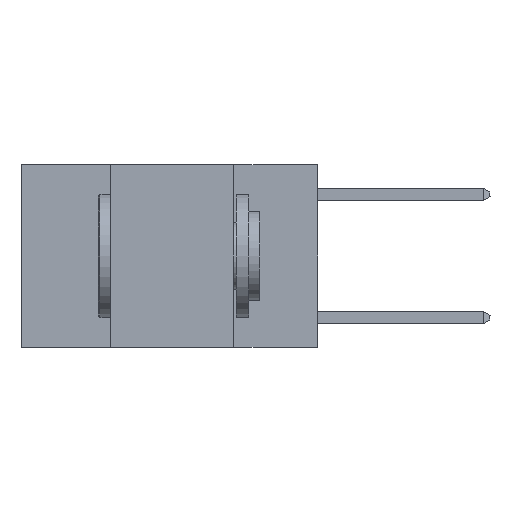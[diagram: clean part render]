
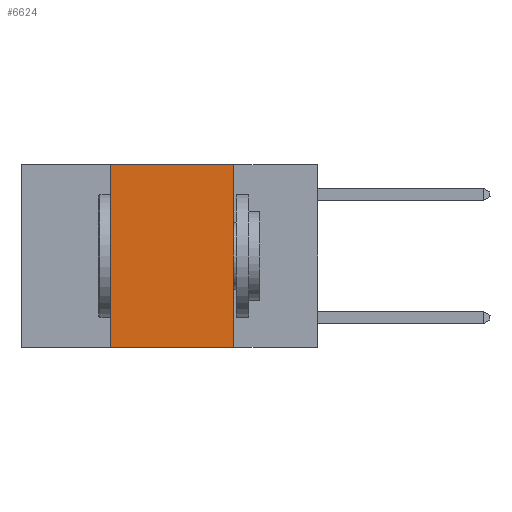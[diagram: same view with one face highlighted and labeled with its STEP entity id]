
A CAD part, left-side view. The second image highlights one B-rep face of the part: STEP entity #6624.
In plain terms, the highlighted planar face has unit normal (-1, 0, 0).
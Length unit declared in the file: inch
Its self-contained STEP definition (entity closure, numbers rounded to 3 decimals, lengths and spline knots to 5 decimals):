
#243 = VERTEX_POINT ( 'NONE', #1435 ) ;
#548 = DIRECTION ( 'NONE',  ( 0., -1., 0. ) ) ;
#835 = LINE ( 'NONE', #12542, #7269 ) ;
#889 = ORIENTED_EDGE ( 'NONE', *, *, #5118, .F. ) ;
#1435 = CARTESIAN_POINT ( 'NONE',  ( 0., 0.17, 0. ) ) ;
#1640 = DIRECTION ( 'NONE',  ( 1., 0., 0. ) ) ;
#1732 = VECTOR ( 'NONE', #548, 39.37008 ) ;
#1780 = LINE ( 'NONE', #12583, #4726 ) ;
#2160 = AXIS2_PLACEMENT_3D ( 'NONE', #2364, #1640, #7473 ) ;
#2265 = CARTESIAN_POINT ( 'NONE',  ( 0., 0.42, 0. ) ) ;
#2364 = CARTESIAN_POINT ( 'NONE',  ( 0., 0.6, 0. ) ) ;
#2411 = EDGE_CURVE ( 'NONE', #8634, #5942, #1780, .T. ) ;
#2758 = LINE ( 'NONE', #9240, #1732 ) ;
#2788 = ORIENTED_EDGE ( 'NONE', *, *, #2411, .T. ) ;
#3867 = DIRECTION ( 'NONE',  ( 0., -1., 0. ) ) ;
#4726 = VECTOR ( 'NONE', #3867, 39.37008 ) ;
#5028 = DIRECTION ( 'NONE',  ( 0., 0., 1. ) ) ;
#5112 = CARTESIAN_POINT ( 'NONE',  ( 0., 0.17, -0.37 ) ) ;
#5118 = EDGE_CURVE ( 'NONE', #8634, #5963, #10957, .T. ) ;
#5543 = EDGE_CURVE ( 'NONE', #5963, #243, #2758, .T. ) ;
#5942 = VERTEX_POINT ( 'NONE', #5112 ) ;
#5963 = VERTEX_POINT ( 'NONE', #6857 ) ;
#5974 = EDGE_CURVE ( 'NONE', #243, #5942, #835, .T. ) ;
#6624 = ADVANCED_FACE ( 'NONE', ( #8160 ), #9246, .F. ) ;
#6857 = CARTESIAN_POINT ( 'NONE',  ( 0., 0.42, 0. ) ) ;
#7269 = VECTOR ( 'NONE', #9650, 39.37008 ) ;
#7473 = DIRECTION ( 'NONE',  ( 0., 0., -1. ) ) ;
#7488 = ORIENTED_EDGE ( 'NONE', *, *, #5974, .F. ) ;
#8160 = FACE_OUTER_BOUND ( 'NONE', #10962, .T. ) ;
#8634 = VERTEX_POINT ( 'NONE', #9545 ) ;
#9240 = CARTESIAN_POINT ( 'NONE',  ( 0., 0.6, 0. ) ) ;
#9246 = PLANE ( 'NONE',  #2160 ) ;
#9545 = CARTESIAN_POINT ( 'NONE',  ( 0., 0.42, -0.37 ) ) ;
#9650 = DIRECTION ( 'NONE',  ( 0., 0., -1. ) ) ;
#10957 = LINE ( 'NONE', #2265, #12402 ) ;
#10962 = EDGE_LOOP ( 'NONE', ( #7488, #12110, #889, #2788 ) ) ;
#12110 = ORIENTED_EDGE ( 'NONE', *, *, #5543, .F. ) ;
#12402 = VECTOR ( 'NONE', #5028, 39.37008 ) ;
#12542 = CARTESIAN_POINT ( 'NONE',  ( 0., 0.17, 0. ) ) ;
#12583 = CARTESIAN_POINT ( 'NONE',  ( 0., 0.6, -0.37 ) ) ;
